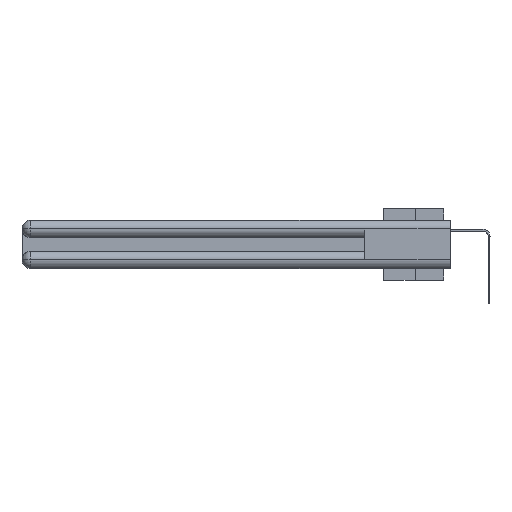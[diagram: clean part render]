
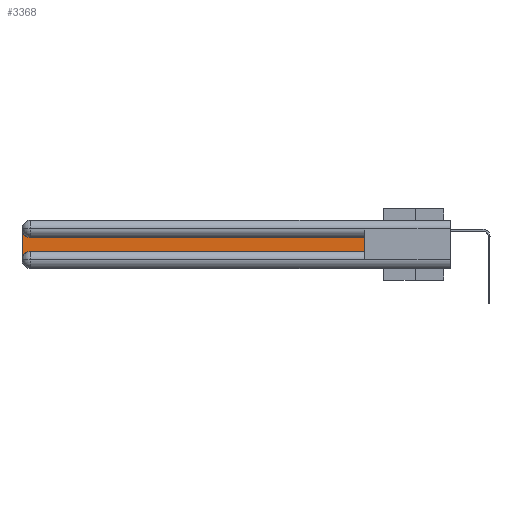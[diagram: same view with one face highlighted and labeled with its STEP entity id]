
A CAD part, left-side view. The second image highlights one B-rep face of the part: STEP entity #3368.
In plain terms, the highlighted planar face has unit normal (-1, 0, 0).
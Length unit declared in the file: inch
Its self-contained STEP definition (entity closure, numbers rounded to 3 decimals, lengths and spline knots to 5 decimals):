
#58 = CARTESIAN_POINT ( 'NONE',  ( 0.075, 2.94, -0.1225 ) ) ;
#708 = VECTOR ( 'NONE', #16153, 39.37008 ) ;
#710 = VECTOR ( 'NONE', #35256, 39.37008 ) ;
#1167 = EDGE_LOOP ( 'NONE', ( #36614, #12289, #12848, #23701, #26061, #24370 ) ) ;
#1440 = VECTOR ( 'NONE', #35231, 39.37008 ) ;
#1789 = EDGE_CURVE ( 'NONE', #11145, #4098, #26117, .T. ) ;
#1801 = CARTESIAN_POINT ( 'NONE',  ( 0.075, 2.94, -0.2175 ) ) ;
#2521 = AXIS2_PLACEMENT_3D ( 'NONE', #15065, #17979, #18105 ) ;
#2818 = VECTOR ( 'NONE', #24996, 39.37008 ) ;
#3368 = ADVANCED_FACE ( 'NONE', ( #36542 ), #32761, .F. ) ;
#3731 = CARTESIAN_POINT ( 'NONE',  ( 0.075, 0.6, -0.2175 ) ) ;
#4098 = VERTEX_POINT ( 'NONE', #33378 ) ;
#5779 = LINE ( 'NONE', #13362, #1440 ) ;
#6060 = AXIS2_PLACEMENT_3D ( 'NONE', #31316, #10292, #34688 ) ;
#9268 = LINE ( 'NONE', #10990, #710 ) ;
#10292 = DIRECTION ( 'NONE',  ( 1., 0., 0. ) ) ;
#10990 = CARTESIAN_POINT ( 'NONE',  ( 0.075, 0.6, -0.2175 ) ) ;
#11145 = VERTEX_POINT ( 'NONE', #25262 ) ;
#12289 = ORIENTED_EDGE ( 'NONE', *, *, #19579, .T. ) ;
#12341 = EDGE_CURVE ( 'NONE', #21488, #21693, #32164, .T. ) ;
#12848 = ORIENTED_EDGE ( 'NONE', *, *, #12341, .T. ) ;
#13362 = CARTESIAN_POINT ( 'NONE',  ( 0.075, 0.6, -0.1225 ) ) ;
#14512 = CARTESIAN_POINT ( 'NONE',  ( 0.075, 3., -0.1225 ) ) ;
#14675 = CIRCLE ( 'NONE', #6060, 0.06 ) ;
#15065 = CARTESIAN_POINT ( 'NONE',  ( 0.075, 2.94, -0.0625 ) ) ;
#16153 = DIRECTION ( 'NONE',  ( 0., 0., -1. ) ) ;
#16165 = CARTESIAN_POINT ( 'NONE',  ( 0.075, 3., -0.0625 ) ) ;
#16904 = VERTEX_POINT ( 'NONE', #1801 ) ;
#17542 = DIRECTION ( 'NONE',  ( 0., 0., -1. ) ) ;
#17791 = EDGE_CURVE ( 'NONE', #4098, #28265, #5779, .T. ) ;
#17979 = DIRECTION ( 'NONE',  ( 1., 0., 0. ) ) ;
#18105 = DIRECTION ( 'NONE',  ( 0., 0., -1. ) ) ;
#19117 = EDGE_CURVE ( 'NONE', #21693, #16904, #14675, .T. ) ;
#19579 = EDGE_CURVE ( 'NONE', #28265, #21488, #25553, .T. ) ;
#21488 = VERTEX_POINT ( 'NONE', #16165 ) ;
#21693 = VERTEX_POINT ( 'NONE', #29372 ) ;
#23372 = DIRECTION ( 'NONE',  ( 1., 0., 0. ) ) ;
#23701 = ORIENTED_EDGE ( 'NONE', *, *, #19117, .T. ) ;
#24370 = ORIENTED_EDGE ( 'NONE', *, *, #1789, .T. ) ;
#24996 = DIRECTION ( 'NONE',  ( 0., 0., 1. ) ) ;
#25005 = EDGE_CURVE ( 'NONE', #16904, #11145, #9268, .T. ) ;
#25262 = CARTESIAN_POINT ( 'NONE',  ( 0.075, 0.6, -0.2175 ) ) ;
#25553 = CIRCLE ( 'NONE', #2521, 0.06 ) ;
#26061 = ORIENTED_EDGE ( 'NONE', *, *, #25005, .T. ) ;
#26117 = LINE ( 'NONE', #3731, #2818 ) ;
#28265 = VERTEX_POINT ( 'NONE', #58 ) ;
#29372 = CARTESIAN_POINT ( 'NONE',  ( 0.075, 3., -0.2775 ) ) ;
#31316 = CARTESIAN_POINT ( 'NONE',  ( 0.075, 2.94, -0.2775 ) ) ;
#32164 = LINE ( 'NONE', #37246, #708 ) ;
#32761 = PLANE ( 'NONE',  #37456 ) ;
#33378 = CARTESIAN_POINT ( 'NONE',  ( 0.075, 0.6, -0.1225 ) ) ;
#34688 = DIRECTION ( 'NONE',  ( 0., 0., -1. ) ) ;
#35231 = DIRECTION ( 'NONE',  ( 0., 1., 0. ) ) ;
#35256 = DIRECTION ( 'NONE',  ( 0., -1., 0. ) ) ;
#36542 = FACE_OUTER_BOUND ( 'NONE', #1167, .T. ) ;
#36614 = ORIENTED_EDGE ( 'NONE', *, *, #17791, .T. ) ;
#37246 = CARTESIAN_POINT ( 'NONE',  ( 0.075, 3., -0.2175 ) ) ;
#37456 = AXIS2_PLACEMENT_3D ( 'NONE', #14512, #23372, #17542 ) ;
